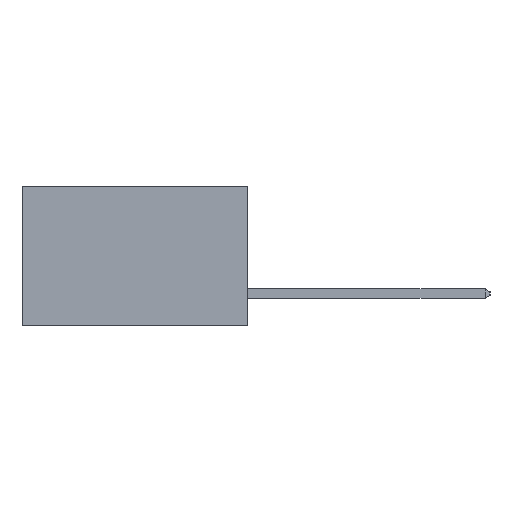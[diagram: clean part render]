
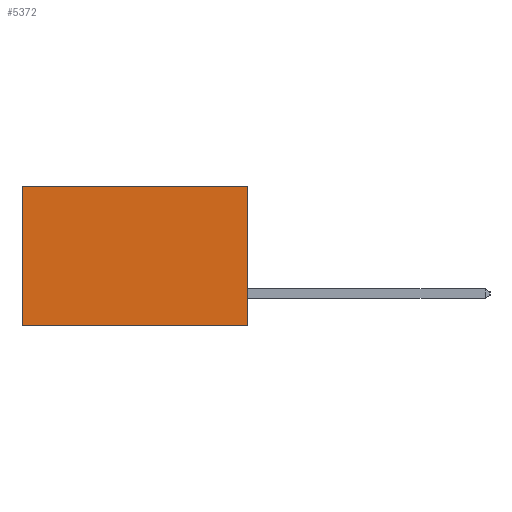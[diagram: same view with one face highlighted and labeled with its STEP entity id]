
A CAD part, left-side view. The second image highlights one B-rep face of the part: STEP entity #5372.
In plain terms, the highlighted planar face has unit normal (-1, 0, 0).
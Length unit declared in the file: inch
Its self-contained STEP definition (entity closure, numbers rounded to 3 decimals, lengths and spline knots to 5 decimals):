
#32 = DIRECTION ( 'NONE',  ( 0., 1., 0. ) ) ;
#294 = CARTESIAN_POINT ( 'NONE',  ( 0.298, 0., 0. ) ) ;
#634 = ORIENTED_EDGE ( 'NONE', *, *, #6829, .F. ) ;
#867 = CARTESIAN_POINT ( 'NONE',  ( 0.298, 0.6, 0. ) ) ;
#1533 = EDGE_LOOP ( 'NONE', ( #3391, #2156, #634, #8071 ) ) ;
#1635 = VECTOR ( 'NONE', #8031, 39.37008 ) ;
#2156 = ORIENTED_EDGE ( 'NONE', *, *, #9151, .F. ) ;
#2246 = EDGE_CURVE ( 'NONE', #8756, #8770, #8148, .T. ) ;
#2582 = DIRECTION ( 'NONE',  ( 0., 0., -1. ) ) ;
#3391 = ORIENTED_EDGE ( 'NONE', *, *, #2246, .T. ) ;
#3714 = VERTEX_POINT ( 'NONE', #294 ) ;
#4361 = VECTOR ( 'NONE', #7871, 39.37008 ) ;
#5284 = VERTEX_POINT ( 'NONE', #9923 ) ;
#5372 = ADVANCED_FACE ( 'NONE', ( #14372 ), #10544, .F. ) ;
#5670 = CARTESIAN_POINT ( 'NONE',  ( 0.298, 0.6, -0.37 ) ) ;
#6542 = EDGE_CURVE ( 'NONE', #3714, #8756, #10735, .T. ) ;
#6829 = EDGE_CURVE ( 'NONE', #3714, #5284, #7994, .T. ) ;
#7871 = DIRECTION ( 'NONE',  ( 0., 0., -1. ) ) ;
#7921 = CARTESIAN_POINT ( 'NONE',  ( 0.298, 0., 0. ) ) ;
#7994 = LINE ( 'NONE', #7921, #4361 ) ;
#8031 = DIRECTION ( 'NONE',  ( 0., 1., 0. ) ) ;
#8071 = ORIENTED_EDGE ( 'NONE', *, *, #6542, .T. ) ;
#8148 = LINE ( 'NONE', #867, #12969 ) ;
#8756 = VERTEX_POINT ( 'NONE', #8871 ) ;
#8770 = VERTEX_POINT ( 'NONE', #5670 ) ;
#8871 = CARTESIAN_POINT ( 'NONE',  ( 0.298, 0.6, 0. ) ) ;
#9144 = CARTESIAN_POINT ( 'NONE',  ( 0.298, 0., 0. ) ) ;
#9151 = EDGE_CURVE ( 'NONE', #5284, #8770, #14152, .T. ) ;
#9614 = DIRECTION ( 'NONE',  ( 0., 0., -1. ) ) ;
#9923 = CARTESIAN_POINT ( 'NONE',  ( 0.298, 0., -0.37 ) ) ;
#10544 = PLANE ( 'NONE',  #12949 ) ;
#10735 = LINE ( 'NONE', #9144, #1635 ) ;
#11487 = VECTOR ( 'NONE', #32, 39.37008 ) ;
#11914 = CARTESIAN_POINT ( 'NONE',  ( 0.298, 0., 0. ) ) ;
#11953 = DIRECTION ( 'NONE',  ( 1., 0., 0. ) ) ;
#12949 = AXIS2_PLACEMENT_3D ( 'NONE', #11914, #11953, #9614 ) ;
#12969 = VECTOR ( 'NONE', #2582, 39.37008 ) ;
#13445 = CARTESIAN_POINT ( 'NONE',  ( 0.298, 0., -0.37 ) ) ;
#14152 = LINE ( 'NONE', #13445, #11487 ) ;
#14372 = FACE_OUTER_BOUND ( 'NONE', #1533, .T. ) ;
